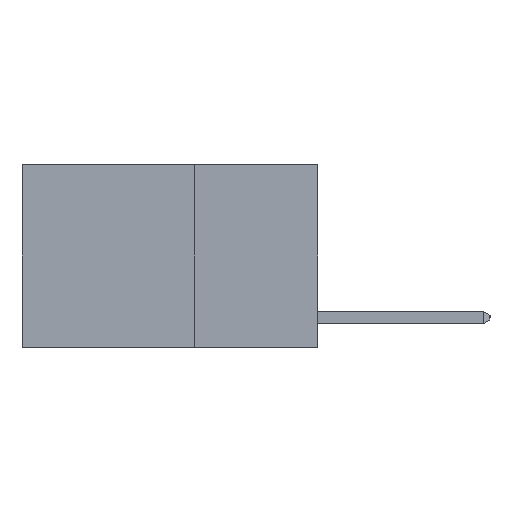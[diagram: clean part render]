
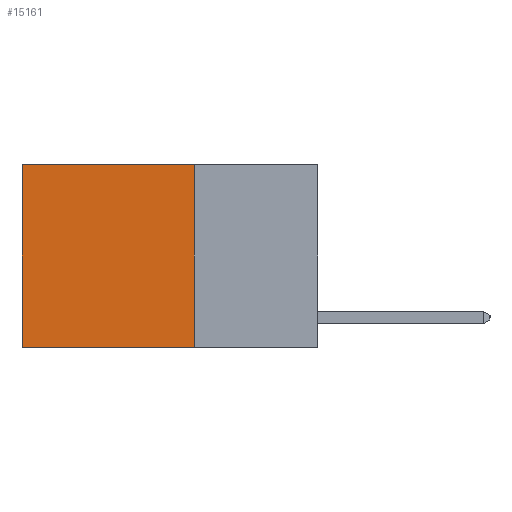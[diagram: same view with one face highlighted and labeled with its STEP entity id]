
A CAD part, left-side view. The second image highlights one B-rep face of the part: STEP entity #15161.
In plain terms, the highlighted planar face has unit normal (-1, 0, 0).
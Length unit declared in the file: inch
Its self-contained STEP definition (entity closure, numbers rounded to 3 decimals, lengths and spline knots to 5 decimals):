
#316 = EDGE_CURVE ( 'NONE', #3568, #2719, #10299, .T. ) ;
#458 = VECTOR ( 'NONE', #13696, 39.37008 ) ;
#654 = ORIENTED_EDGE ( 'NONE', *, *, #5789, .T. ) ;
#873 = CARTESIAN_POINT ( 'NONE',  ( 0.2625, 0.25, 0. ) ) ;
#1100 = EDGE_CURVE ( 'NONE', #1379, #5234, #9270, .T. ) ;
#1379 = VERTEX_POINT ( 'NONE', #11668 ) ;
#2405 = PLANE ( 'NONE',  #9205 ) ;
#2719 = VERTEX_POINT ( 'NONE', #9765 ) ;
#3568 = VERTEX_POINT ( 'NONE', #3701 ) ;
#3701 = CARTESIAN_POINT ( 'NONE',  ( 0.2625, 0.25, 0. ) ) ;
#3942 = LINE ( 'NONE', #7271, #6944 ) ;
#5234 = VERTEX_POINT ( 'NONE', #13717 ) ;
#5265 = VECTOR ( 'NONE', #6089, 39.37008 ) ;
#5789 = EDGE_CURVE ( 'NONE', #2719, #5234, #3942, .T. ) ;
#6089 = DIRECTION ( 'NONE',  ( 0., 0., -1. ) ) ;
#6150 = DIRECTION ( 'NONE',  ( 0., 1., 0. ) ) ;
#6366 = ORIENTED_EDGE ( 'NONE', *, *, #1100, .F. ) ;
#6944 = VECTOR ( 'NONE', #9793, 39.37008 ) ;
#7271 = CARTESIAN_POINT ( 'NONE',  ( 0.2625, 0.6, 0. ) ) ;
#7572 = DIRECTION ( 'NONE',  ( 1., 0., 0. ) ) ;
#7939 = ORIENTED_EDGE ( 'NONE', *, *, #316, .T. ) ;
#8778 = EDGE_CURVE ( 'NONE', #3568, #1379, #15286, .T. ) ;
#9205 = AXIS2_PLACEMENT_3D ( 'NONE', #15074, #7572, #16246 ) ;
#9270 = LINE ( 'NONE', #13519, #12298 ) ;
#9572 = CARTESIAN_POINT ( 'NONE',  ( 0.2625, 0.25, 0. ) ) ;
#9765 = CARTESIAN_POINT ( 'NONE',  ( 0.2625, 0.6, 0. ) ) ;
#9793 = DIRECTION ( 'NONE',  ( 0., 0., -1. ) ) ;
#10299 = LINE ( 'NONE', #9572, #458 ) ;
#11668 = CARTESIAN_POINT ( 'NONE',  ( 0.2625, 0.25, -0.37 ) ) ;
#11769 = EDGE_LOOP ( 'NONE', ( #654, #6366, #15403, #7939 ) ) ;
#12135 = FACE_OUTER_BOUND ( 'NONE', #11769, .T. ) ;
#12298 = VECTOR ( 'NONE', #6150, 39.37008 ) ;
#13519 = CARTESIAN_POINT ( 'NONE',  ( 0.2625, 0.25, -0.37 ) ) ;
#13696 = DIRECTION ( 'NONE',  ( 0., 1., 0. ) ) ;
#13717 = CARTESIAN_POINT ( 'NONE',  ( 0.2625, 0.6, -0.37 ) ) ;
#15074 = CARTESIAN_POINT ( 'NONE',  ( 0.2625, 0.25, 0. ) ) ;
#15161 = ADVANCED_FACE ( 'NONE', ( #12135 ), #2405, .F. ) ;
#15286 = LINE ( 'NONE', #873, #5265 ) ;
#15403 = ORIENTED_EDGE ( 'NONE', *, *, #8778, .F. ) ;
#16246 = DIRECTION ( 'NONE',  ( 0., 0., -1. ) ) ;
